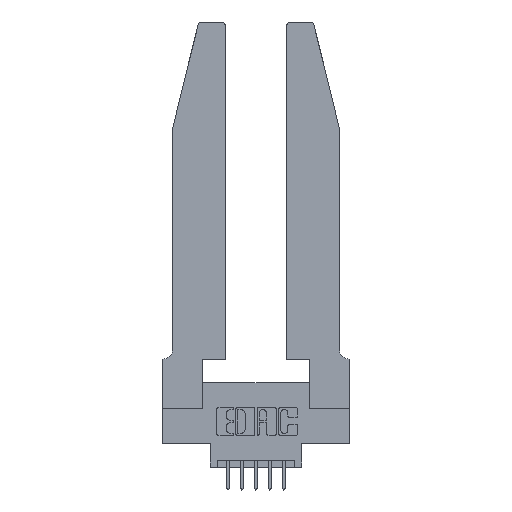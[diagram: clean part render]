
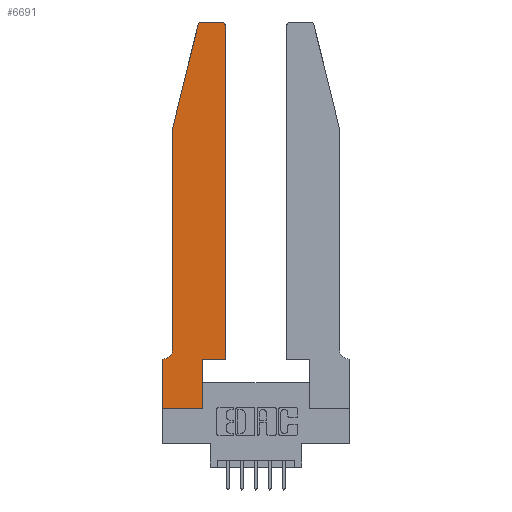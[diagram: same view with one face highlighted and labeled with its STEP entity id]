
A CAD part, top view. The second image highlights one B-rep face of the part: STEP entity #6691.
In plain terms, the highlighted planar face has unit normal (0, 0, 1).
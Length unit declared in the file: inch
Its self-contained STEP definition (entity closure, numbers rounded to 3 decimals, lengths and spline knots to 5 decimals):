
#228 = EDGE_CURVE ( 'NONE', #7639, #5718, #9060, .T. ) ;
#359 = DIRECTION ( 'NONE',  ( -1., 0., 0. ) ) ;
#634 = CARTESIAN_POINT ( 'NONE',  ( 0.2865, 0., 0.37 ) ) ;
#718 = LINE ( 'NONE', #10994, #4247 ) ;
#793 = DIRECTION ( 'NONE',  ( 0., -1., 0. ) ) ;
#837 = LINE ( 'NONE', #13489, #12729 ) ;
#1207 = VECTOR ( 'NONE', #4200, 39.37008 ) ;
#1319 = CARTESIAN_POINT ( 'NONE',  ( 0., 0.35, 0.37 ) ) ;
#1814 = EDGE_CURVE ( 'NONE', #10985, #7639, #4110, .T. ) ;
#1873 = EDGE_CURVE ( 'NONE', #6709, #3309, #5283, .T. ) ;
#2142 = DIRECTION ( 'NONE',  ( -1., 0., 0. ) ) ;
#2196 = EDGE_LOOP ( 'NONE', ( #11168, #8739, #12610, #4409, #9549, #10528, #8085, #11591, #2493, #8123, #8159, #10471 ) ) ;
#2292 = DIRECTION ( 'NONE',  ( 0., 0., 1. ) ) ;
#2493 = ORIENTED_EDGE ( 'NONE', *, *, #5448, .T. ) ;
#2581 = VERTEX_POINT ( 'NONE', #7137 ) ;
#2730 = CARTESIAN_POINT ( 'NONE',  ( 0.0755, 2., 0.37 ) ) ;
#3079 = CARTESIAN_POINT ( 'NONE',  ( 0.0755, 0.35, 0.37 ) ) ;
#3309 = VERTEX_POINT ( 'NONE', #9741 ) ;
#3512 = PLANE ( 'NONE',  #12996 ) ;
#3861 = VERTEX_POINT ( 'NONE', #634 ) ;
#3921 = DIRECTION ( 'NONE',  ( 0., -1., 0. ) ) ;
#4110 = CIRCLE ( 'NONE', #6588, 0.07 ) ;
#4177 = VECTOR ( 'NONE', #2142, 39.37008 ) ;
#4200 = DIRECTION ( 'NONE',  ( -1., 0., 0. ) ) ;
#4247 = VECTOR ( 'NONE', #8957, 39.37008 ) ;
#4409 = ORIENTED_EDGE ( 'NONE', *, *, #11827, .T. ) ;
#4537 = VERTEX_POINT ( 'NONE', #6155 ) ;
#4572 = AXIS2_PLACEMENT_3D ( 'NONE', #9724, #6656, #6696 ) ;
#4729 = DIRECTION ( 'NONE',  ( 0., 0., 1. ) ) ;
#4947 = CARTESIAN_POINT ( 'NONE',  ( 0., 0.35, 0.37 ) ) ;
#5283 = LINE ( 'NONE', #13443, #9107 ) ;
#5339 = EDGE_CURVE ( 'NONE', #4537, #2581, #12387, .T. ) ;
#5435 = LINE ( 'NONE', #9234, #11452 ) ;
#5448 = EDGE_CURVE ( 'NONE', #3861, #6709, #837, .T. ) ;
#5499 = CIRCLE ( 'NONE', #12668, 0.03 ) ;
#5718 = VERTEX_POINT ( 'NONE', #4947 ) ;
#5887 = CARTESIAN_POINT ( 'NONE',  ( 0.0755, 0.42, 0.37 ) ) ;
#6034 = DIRECTION ( 'NONE',  ( 0., 1., 0. ) ) ;
#6155 = CARTESIAN_POINT ( 'NONE',  ( 0.4505, 2.72, 0.37 ) ) ;
#6180 = VERTEX_POINT ( 'NONE', #2730 ) ;
#6540 = EDGE_CURVE ( 'NONE', #2581, #11718, #9006, .T. ) ;
#6588 = AXIS2_PLACEMENT_3D ( 'NONE', #10982, #13115, #359 ) ;
#6591 = EDGE_CURVE ( 'NONE', #12407, #6180, #10357, .T. ) ;
#6656 = DIRECTION ( 'NONE',  ( 0., 0., 1. ) ) ;
#6691 = ADVANCED_FACE ( 'NONE', ( #12858 ), #3512, .T. ) ;
#6696 = DIRECTION ( 'NONE',  ( 1., 0., 0. ) ) ;
#6709 = VERTEX_POINT ( 'NONE', #13102 ) ;
#7137 = CARTESIAN_POINT ( 'NONE',  ( 0.4205, 2.75, 0.37 ) ) ;
#7195 = CARTESIAN_POINT ( 'NONE',  ( 0., 0., 0.37 ) ) ;
#7517 = VECTOR ( 'NONE', #9883, 39.37008 ) ;
#7639 = VERTEX_POINT ( 'NONE', #12243 ) ;
#7644 = LINE ( 'NONE', #7195, #10830 ) ;
#7764 = EDGE_CURVE ( 'NONE', #5718, #8583, #7644, .T. ) ;
#8085 = ORIENTED_EDGE ( 'NONE', *, *, #7764, .T. ) ;
#8123 = ORIENTED_EDGE ( 'NONE', *, *, #1873, .T. ) ;
#8159 = ORIENTED_EDGE ( 'NONE', *, *, #12750, .T. ) ;
#8295 = CARTESIAN_POINT ( 'NONE',  ( 0.284, 2.75, 0.37 ) ) ;
#8462 = VECTOR ( 'NONE', #12630, 39.37008 ) ;
#8583 = VERTEX_POINT ( 'NONE', #12840 ) ;
#8739 = ORIENTED_EDGE ( 'NONE', *, *, #9793, .T. ) ;
#8957 = DIRECTION ( 'NONE',  ( 0., 1., 0. ) ) ;
#9006 = LINE ( 'NONE', #11690, #4177 ) ;
#9060 = LINE ( 'NONE', #3079, #1207 ) ;
#9107 = VECTOR ( 'NONE', #11713, 39.37008 ) ;
#9234 = CARTESIAN_POINT ( 'NONE',  ( 0.0755, 2., 0.37 ) ) ;
#9549 = ORIENTED_EDGE ( 'NONE', *, *, #1814, .T. ) ;
#9724 = CARTESIAN_POINT ( 'NONE',  ( 0.4205, 2.72, 0.37 ) ) ;
#9741 = CARTESIAN_POINT ( 'NONE',  ( 0.4505, 0.35, 0.37 ) ) ;
#9793 = EDGE_CURVE ( 'NONE', #11718, #12407, #5499, .T. ) ;
#9883 = DIRECTION ( 'NONE',  ( -0.239, -0.971, 0. ) ) ;
#10233 = EDGE_CURVE ( 'NONE', #8583, #3861, #12321, .T. ) ;
#10357 = LINE ( 'NONE', #11937, #7517 ) ;
#10471 = ORIENTED_EDGE ( 'NONE', *, *, #5339, .T. ) ;
#10528 = ORIENTED_EDGE ( 'NONE', *, *, #228, .T. ) ;
#10830 = VECTOR ( 'NONE', #793, 39.37008 ) ;
#10982 = CARTESIAN_POINT ( 'NONE',  ( 0.0055, 0.42, 0.37 ) ) ;
#10985 = VERTEX_POINT ( 'NONE', #5887 ) ;
#10994 = CARTESIAN_POINT ( 'NONE',  ( 0.4505, 0.35, 0.37 ) ) ;
#11092 = DIRECTION ( 'NONE',  ( 1., 0., 0. ) ) ;
#11168 = ORIENTED_EDGE ( 'NONE', *, *, #6540, .T. ) ;
#11452 = VECTOR ( 'NONE', #3921, 39.37008 ) ;
#11591 = ORIENTED_EDGE ( 'NONE', *, *, #10233, .T. ) ;
#11690 = CARTESIAN_POINT ( 'NONE',  ( 0.2605, 2.75, 0.37 ) ) ;
#11713 = DIRECTION ( 'NONE',  ( 1., 0., 0. ) ) ;
#11718 = VERTEX_POINT ( 'NONE', #8295 ) ;
#11827 = EDGE_CURVE ( 'NONE', #6180, #10985, #5435, .T. ) ;
#11830 = CARTESIAN_POINT ( 'NONE',  ( 0.284, 2.72, 0.37 ) ) ;
#11937 = CARTESIAN_POINT ( 'NONE',  ( 0.0755, 2., 0.37 ) ) ;
#12117 = DIRECTION ( 'NONE',  ( 1., 0., 0. ) ) ;
#12243 = CARTESIAN_POINT ( 'NONE',  ( 0.0055, 0.35, 0.37 ) ) ;
#12321 = LINE ( 'NONE', #13849, #8462 ) ;
#12387 = CIRCLE ( 'NONE', #4572, 0.03 ) ;
#12407 = VERTEX_POINT ( 'NONE', #13796 ) ;
#12610 = ORIENTED_EDGE ( 'NONE', *, *, #6591, .T. ) ;
#12630 = DIRECTION ( 'NONE',  ( 1., 0., 0. ) ) ;
#12668 = AXIS2_PLACEMENT_3D ( 'NONE', #11830, #4729, #11092 ) ;
#12729 = VECTOR ( 'NONE', #6034, 39.37008 ) ;
#12750 = EDGE_CURVE ( 'NONE', #3309, #4537, #718, .T. ) ;
#12840 = CARTESIAN_POINT ( 'NONE',  ( 0., 0., 0.37 ) ) ;
#12858 = FACE_OUTER_BOUND ( 'NONE', #2196, .T. ) ;
#12996 = AXIS2_PLACEMENT_3D ( 'NONE', #1319, #2292, #12117 ) ;
#13102 = CARTESIAN_POINT ( 'NONE',  ( 0.2865, 0.35, 0.37 ) ) ;
#13115 = DIRECTION ( 'NONE',  ( 0., 0., -1. ) ) ;
#13443 = CARTESIAN_POINT ( 'NONE',  ( 0.4505, 0.35, 0.37 ) ) ;
#13489 = CARTESIAN_POINT ( 'NONE',  ( 0.2865, 0.35, 0.37 ) ) ;
#13796 = CARTESIAN_POINT ( 'NONE',  ( 0.25487, 2.72718, 0.37 ) ) ;
#13849 = CARTESIAN_POINT ( 'NONE',  ( 0., 0., 0.37 ) ) ;
